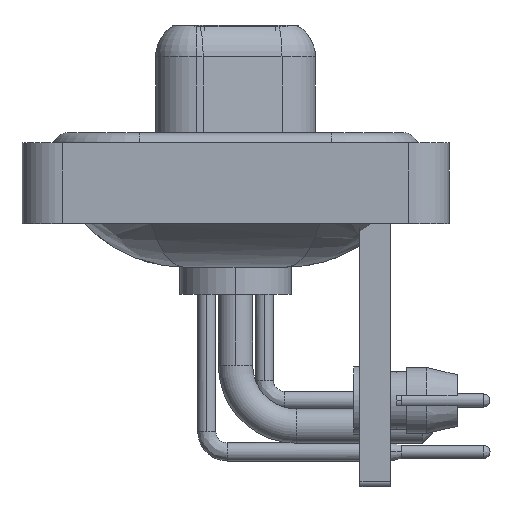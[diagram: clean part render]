
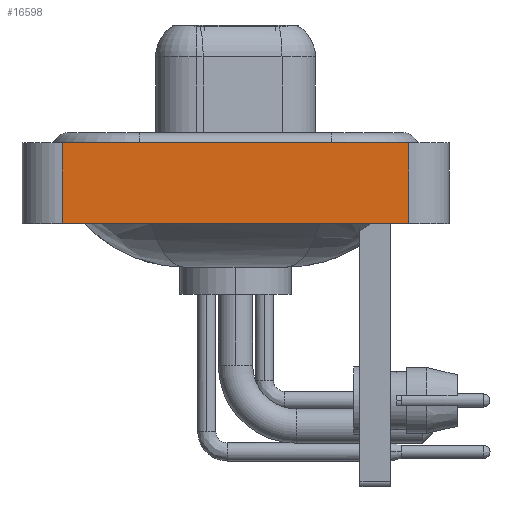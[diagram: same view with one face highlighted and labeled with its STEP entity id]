
A CAD part, left-side view. The second image highlights one B-rep face of the part: STEP entity #16598.
In plain terms, the highlighted planar face has unit normal (-1, 0, 0).
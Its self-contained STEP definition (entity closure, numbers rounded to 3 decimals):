
#1677 = CARTESIAN_POINT ( 'NONE',  ( -7.35, -8.55, 0.4 ) ) ;
#2769 = CARTESIAN_POINT ( 'NONE',  ( -7.35, -8.55, 0.4 ) ) ;
#3352 = DIRECTION ( 'NONE',  ( -1., 0., 0. ) ) ;
#3767 = ORIENTED_EDGE ( 'NONE', *, *, #19946, .T. ) ;
#4046 = CARTESIAN_POINT ( 'NONE',  ( -7.35, -8.55, -3.6 ) ) ;
#4679 = EDGE_CURVE ( 'NONE', #20343, #8196, #6737, .T. ) ;
#5931 = VERTEX_POINT ( 'NONE', #2769 ) ;
#6137 = VERTEX_POINT ( 'NONE', #8588 ) ;
#6737 = LINE ( 'NONE', #8404, #6773 ) ;
#6773 = VECTOR ( 'NONE', #22950, 1000. ) ;
#7152 = CARTESIAN_POINT ( 'NONE',  ( -7.35, -8.55, -3.6 ) ) ;
#7522 = AXIS2_PLACEMENT_3D ( 'NONE', #7152, #3352, #14443 ) ;
#8196 = VERTEX_POINT ( 'NONE', #4046 ) ;
#8258 = DIRECTION ( 'NONE',  ( 0., 0., 1. ) ) ;
#8404 = CARTESIAN_POINT ( 'NONE',  ( -7.35, -8.55, -3.6 ) ) ;
#8588 = CARTESIAN_POINT ( 'NONE',  ( -7.35, 8.55, 0.4 ) ) ;
#10210 = VECTOR ( 'NONE', #19679, 1000. ) ;
#11585 = ORIENTED_EDGE ( 'NONE', *, *, #4679, .T. ) ;
#11667 = CARTESIAN_POINT ( 'NONE',  ( -7.35, -8.55, -3.6 ) ) ;
#12413 = EDGE_CURVE ( 'NONE', #20343, #6137, #13763, .T. ) ;
#12435 = VECTOR ( 'NONE', #8258, 1000. ) ;
#13763 = LINE ( 'NONE', #22565, #12435 ) ;
#14328 = LINE ( 'NONE', #1677, #10210 ) ;
#14443 = DIRECTION ( 'NONE',  ( 0., 0., 1. ) ) ;
#15255 = LINE ( 'NONE', #11667, #20499 ) ;
#16558 = EDGE_CURVE ( 'NONE', #6137, #5931, #14328, .T. ) ;
#16598 = ADVANCED_FACE ( 'NONE', ( #20142 ), #23477, .T. ) ;
#17270 = DIRECTION ( 'NONE',  ( 0., 0., 1. ) ) ;
#18531 = EDGE_LOOP ( 'NONE', ( #3767, #20770, #19479, #11585 ) ) ;
#19479 = ORIENTED_EDGE ( 'NONE', *, *, #12413, .F. ) ;
#19679 = DIRECTION ( 'NONE',  ( 0., -1., 0. ) ) ;
#19816 = CARTESIAN_POINT ( 'NONE',  ( -7.35, 8.55, -3.6 ) ) ;
#19946 = EDGE_CURVE ( 'NONE', #8196, #5931, #15255, .T. ) ;
#20142 = FACE_OUTER_BOUND ( 'NONE', #18531, .T. ) ;
#20343 = VERTEX_POINT ( 'NONE', #19816 ) ;
#20499 = VECTOR ( 'NONE', #17270, 1000. ) ;
#20770 = ORIENTED_EDGE ( 'NONE', *, *, #16558, .F. ) ;
#22565 = CARTESIAN_POINT ( 'NONE',  ( -7.35, 8.55, -3.6 ) ) ;
#22950 = DIRECTION ( 'NONE',  ( 0., -1., 0. ) ) ;
#23477 = PLANE ( 'NONE',  #7522 ) ;
